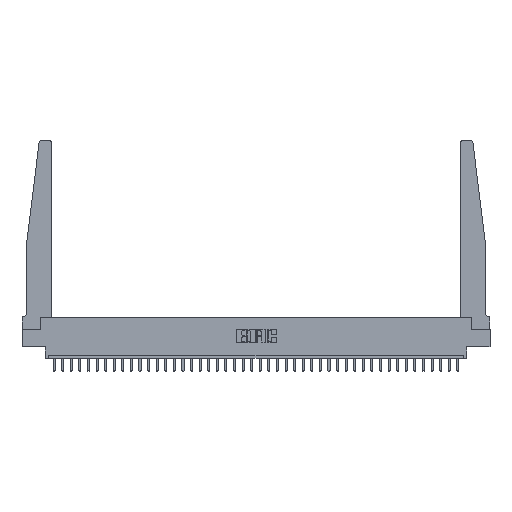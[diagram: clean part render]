
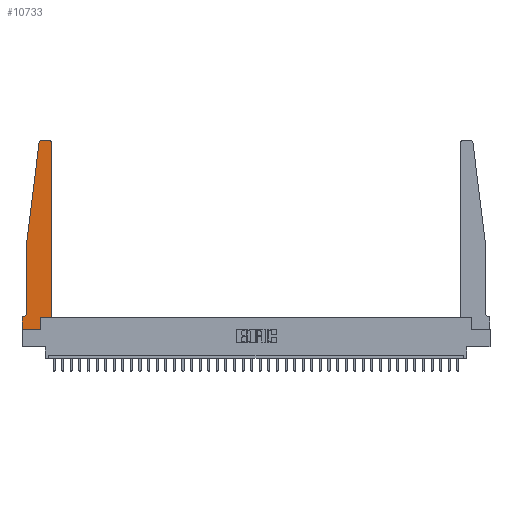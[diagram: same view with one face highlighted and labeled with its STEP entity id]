
A CAD part, top view. The second image highlights one B-rep face of the part: STEP entity #10733.
In plain terms, the highlighted planar face has unit normal (0, 0, 1).
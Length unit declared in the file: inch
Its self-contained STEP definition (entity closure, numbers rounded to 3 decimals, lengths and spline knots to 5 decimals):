
#191 = LINE ( 'NONE', #2973, #33165 ) ;
#1174 = DIRECTION ( 'NONE',  ( 0., 1., 0. ) ) ;
#1265 = CARTESIAN_POINT ( 'NONE',  ( 0., 0.1875, 0.37 ) ) ;
#1696 = ORIENTED_EDGE ( 'NONE', *, *, #16480, .T. ) ;
#1829 = ORIENTED_EDGE ( 'NONE', *, *, #5574, .T. ) ;
#2092 = CARTESIAN_POINT ( 'NONE',  ( 0., 0.1875, 0.37 ) ) ;
#2973 = CARTESIAN_POINT ( 'NONE',  ( 0.425, 0.18, 0.37 ) ) ;
#3025 = AXIS2_PLACEMENT_3D ( 'NONE', #22293, #11608, #19328 ) ;
#3050 = VERTEX_POINT ( 'NONE', #4114 ) ;
#3502 = LINE ( 'NONE', #14003, #28272 ) ;
#3544 = VECTOR ( 'NONE', #29996, 39.37008 ) ;
#3682 = CARTESIAN_POINT ( 'NONE',  ( 0.065, 1.25, 0.37 ) ) ;
#3707 = CIRCLE ( 'NONE', #33144, 0.03 ) ;
#4114 = CARTESIAN_POINT ( 'NONE',  ( 0.27653, 2.75, 0.37 ) ) ;
#4638 = ORIENTED_EDGE ( 'NONE', *, *, #29398, .T. ) ;
#5574 = EDGE_CURVE ( 'NONE', #30541, #25010, #3707, .T. ) ;
#6237 = EDGE_CURVE ( 'NONE', #9960, #29952, #191, .T. ) ;
#6277 = CARTESIAN_POINT ( 'NONE',  ( 0.015, 0.1875, 0.37 ) ) ;
#6637 = DIRECTION ( 'NONE',  ( 1., 0., 0. ) ) ;
#6737 = DIRECTION ( 'NONE',  ( 1., 0., 0. ) ) ;
#7014 = DIRECTION ( 'NONE',  ( -1., 0., 0. ) ) ;
#7601 = CARTESIAN_POINT ( 'NONE',  ( 0.2605, 0., 0.37 ) ) ;
#7638 = DIRECTION ( 'NONE',  ( 0., 0., 1. ) ) ;
#7713 = VERTEX_POINT ( 'NONE', #32225 ) ;
#7807 = ORIENTED_EDGE ( 'NONE', *, *, #32356, .T. ) ;
#8187 = ORIENTED_EDGE ( 'NONE', *, *, #6237, .T. ) ;
#8498 = LINE ( 'NONE', #16459, #30119 ) ;
#9551 = CARTESIAN_POINT ( 'NONE',  ( 0.395, 2.72, 0.37 ) ) ;
#9652 = CIRCLE ( 'NONE', #3025, 0.05 ) ;
#9960 = VERTEX_POINT ( 'NONE', #31638 ) ;
#10064 = CARTESIAN_POINT ( 'NONE',  ( 0.395, 2.75, 0.37 ) ) ;
#10065 = CARTESIAN_POINT ( 'NONE',  ( 0.425, 0.18, 0.37 ) ) ;
#10733 = ADVANCED_FACE ( 'NONE', ( #17872 ), #15243, .T. ) ;
#11608 = DIRECTION ( 'NONE',  ( 0., 0., -1. ) ) ;
#11838 = CIRCLE ( 'NONE', #23591, 0.03 ) ;
#11843 = CARTESIAN_POINT ( 'NONE',  ( 0.25, 2.75, 0.37 ) ) ;
#12101 = ORIENTED_EDGE ( 'NONE', *, *, #29078, .T. ) ;
#12170 = CARTESIAN_POINT ( 'NONE',  ( 0.065, 0.1875, 0.37 ) ) ;
#12640 = DIRECTION ( 'NONE',  ( 0., 0., 1. ) ) ;
#12713 = ORIENTED_EDGE ( 'NONE', *, *, #27486, .T. ) ;
#12817 = VECTOR ( 'NONE', #33259, 39.37008 ) ;
#13162 = VERTEX_POINT ( 'NONE', #20931 ) ;
#14003 = CARTESIAN_POINT ( 'NONE',  ( 0., 0., 0.37 ) ) ;
#14006 = VECTOR ( 'NONE', #7014, 39.37008 ) ;
#14042 = DIRECTION ( 'NONE',  ( 0., 0., 1. ) ) ;
#14423 = EDGE_CURVE ( 'NONE', #15901, #7713, #8498, .T. ) ;
#14619 = EDGE_CURVE ( 'NONE', #13162, #15901, #25082, .T. ) ;
#14856 = LINE ( 'NONE', #33569, #17706 ) ;
#15243 = PLANE ( 'NONE',  #18859 ) ;
#15901 = VERTEX_POINT ( 'NONE', #3682 ) ;
#15917 = EDGE_CURVE ( 'NONE', #27351, #32994, #3502, .T. ) ;
#16334 = ORIENTED_EDGE ( 'NONE', *, *, #15917, .T. ) ;
#16459 = CARTESIAN_POINT ( 'NONE',  ( 0.065, 1.25, 0.37 ) ) ;
#16480 = EDGE_CURVE ( 'NONE', #22911, #9960, #27988, .T. ) ;
#16910 = CARTESIAN_POINT ( 'NONE',  ( 0.425, 2.72, 0.37 ) ) ;
#17706 = VECTOR ( 'NONE', #6737, 39.37008 ) ;
#17872 = FACE_OUTER_BOUND ( 'NONE', #30618, .T. ) ;
#18315 = EDGE_CURVE ( 'NONE', #29952, #30541, #27358, .T. ) ;
#18493 = VERTEX_POINT ( 'NONE', #6277 ) ;
#18591 = CARTESIAN_POINT ( 'NONE',  ( 0., 0., 0.37 ) ) ;
#18859 = AXIS2_PLACEMENT_3D ( 'NONE', #2092, #12640, #31341 ) ;
#18991 = ORIENTED_EDGE ( 'NONE', *, *, #14619, .T. ) ;
#19328 = DIRECTION ( 'NONE',  ( -1., 0., 0. ) ) ;
#20798 = VECTOR ( 'NONE', #27613, 39.37008 ) ;
#20888 = CARTESIAN_POINT ( 'NONE',  ( 0.27653, 2.72, 0.37 ) ) ;
#20931 = CARTESIAN_POINT ( 'NONE',  ( 0.24675, 2.72367, 0.37 ) ) ;
#21726 = EDGE_CURVE ( 'NONE', #32994, #22911, #14856, .T. ) ;
#22293 = CARTESIAN_POINT ( 'NONE',  ( 0.015, 0.2375, 0.37 ) ) ;
#22623 = CARTESIAN_POINT ( 'NONE',  ( 0.065, 1.25, 0.37 ) ) ;
#22711 = LINE ( 'NONE', #11843, #20798 ) ;
#22911 = VERTEX_POINT ( 'NONE', #7601 ) ;
#23181 = ORIENTED_EDGE ( 'NONE', *, *, #14423, .T. ) ;
#23591 = AXIS2_PLACEMENT_3D ( 'NONE', #20888, #7638, #31698 ) ;
#24560 = DIRECTION ( 'NONE',  ( 0., -1., 0. ) ) ;
#24979 = LINE ( 'NONE', #12170, #14006 ) ;
#25010 = VERTEX_POINT ( 'NONE', #10064 ) ;
#25049 = CARTESIAN_POINT ( 'NONE',  ( 0.2605, 0.18, 0.37 ) ) ;
#25082 = LINE ( 'NONE', #22623, #12817 ) ;
#25410 = ORIENTED_EDGE ( 'NONE', *, *, #18315, .T. ) ;
#27036 = CARTESIAN_POINT ( 'NONE',  ( 0.425, 0.18, 0.37 ) ) ;
#27351 = VERTEX_POINT ( 'NONE', #1265 ) ;
#27358 = LINE ( 'NONE', #27036, #3544 ) ;
#27486 = EDGE_CURVE ( 'NONE', #3050, #13162, #11838, .T. ) ;
#27613 = DIRECTION ( 'NONE',  ( -1., 0., 0. ) ) ;
#27988 = LINE ( 'NONE', #25049, #31925 ) ;
#28216 = ORIENTED_EDGE ( 'NONE', *, *, #21726, .T. ) ;
#28272 = VECTOR ( 'NONE', #30829, 39.37008 ) ;
#28282 = DIRECTION ( 'NONE',  ( 1., 0., 0. ) ) ;
#29078 = EDGE_CURVE ( 'NONE', #7713, #18493, #9652, .T. ) ;
#29398 = EDGE_CURVE ( 'NONE', #25010, #3050, #22711, .T. ) ;
#29952 = VERTEX_POINT ( 'NONE', #10065 ) ;
#29996 = DIRECTION ( 'NONE',  ( 0., 1., 0. ) ) ;
#30119 = VECTOR ( 'NONE', #24560, 39.37008 ) ;
#30541 = VERTEX_POINT ( 'NONE', #16910 ) ;
#30618 = EDGE_LOOP ( 'NONE', ( #4638, #12713, #18991, #23181, #12101, #7807, #16334, #28216, #1696, #8187, #25410, #1829 ) ) ;
#30829 = DIRECTION ( 'NONE',  ( 0., -1., 0. ) ) ;
#31341 = DIRECTION ( 'NONE',  ( 1., 0., 0. ) ) ;
#31638 = CARTESIAN_POINT ( 'NONE',  ( 0.2605, 0.18, 0.37 ) ) ;
#31698 = DIRECTION ( 'NONE',  ( 1., 0., 0. ) ) ;
#31925 = VECTOR ( 'NONE', #1174, 39.37008 ) ;
#32225 = CARTESIAN_POINT ( 'NONE',  ( 0.065, 0.2375, 0.37 ) ) ;
#32356 = EDGE_CURVE ( 'NONE', #18493, #27351, #24979, .T. ) ;
#32994 = VERTEX_POINT ( 'NONE', #18591 ) ;
#33144 = AXIS2_PLACEMENT_3D ( 'NONE', #9551, #14042, #6637 ) ;
#33165 = VECTOR ( 'NONE', #28282, 39.37008 ) ;
#33259 = DIRECTION ( 'NONE',  ( -0.122, -0.992, 0. ) ) ;
#33569 = CARTESIAN_POINT ( 'NONE',  ( 0., 0., 0.37 ) ) ;
